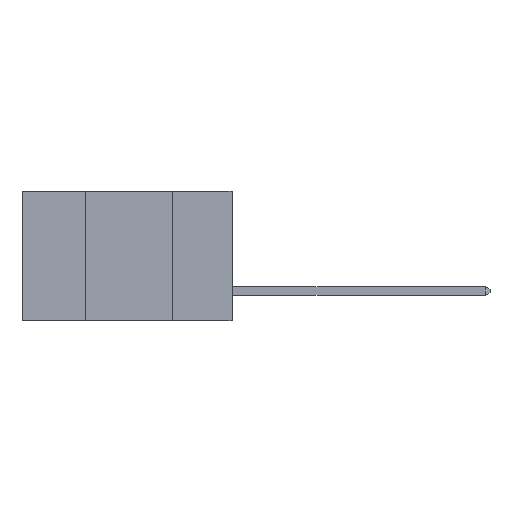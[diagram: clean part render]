
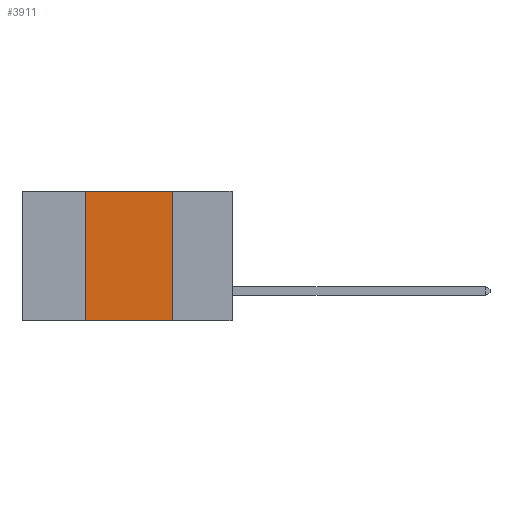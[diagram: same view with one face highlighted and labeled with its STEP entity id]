
A CAD part, left-side view. The second image highlights one B-rep face of the part: STEP entity #3911.
In plain terms, the highlighted planar face has unit normal (-1, 0, 0).
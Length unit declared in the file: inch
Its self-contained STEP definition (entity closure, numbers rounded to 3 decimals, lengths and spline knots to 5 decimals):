
#814 = VERTEX_POINT ( 'NONE', #1011 ) ;
#937 = CARTESIAN_POINT ( 'NONE',  ( 0., 0.42, -0.37 ) ) ;
#1011 = CARTESIAN_POINT ( 'NONE',  ( 0., 0.17, -0.37 ) ) ;
#1382 = VECTOR ( 'NONE', #5724, 39.37008 ) ;
#1448 = VERTEX_POINT ( 'NONE', #6835 ) ;
#3547 = VERTEX_POINT ( 'NONE', #10674 ) ;
#3552 = LINE ( 'NONE', #11912, #1382 ) ;
#3763 = FACE_OUTER_BOUND ( 'NONE', #13095, .T. ) ;
#3911 = ADVANCED_FACE ( 'NONE', ( #3763 ), #10203, .F. ) ;
#3932 = CARTESIAN_POINT ( 'NONE',  ( 0., 0.6, 0. ) ) ;
#3969 = CARTESIAN_POINT ( 'NONE',  ( 0., 0.17, 0. ) ) ;
#4545 = EDGE_CURVE ( 'NONE', #1448, #814, #10468, .T. ) ;
#4776 = LINE ( 'NONE', #7446, #13009 ) ;
#5025 = DIRECTION ( 'NONE',  ( 1., 0., 0. ) ) ;
#5724 = DIRECTION ( 'NONE',  ( 0., -1., 0. ) ) ;
#5783 = CARTESIAN_POINT ( 'NONE',  ( 0., 0.42, 0. ) ) ;
#5859 = ORIENTED_EDGE ( 'NONE', *, *, #4545, .F. ) ;
#6835 = CARTESIAN_POINT ( 'NONE',  ( 0., 0.17, 0. ) ) ;
#7157 = ORIENTED_EDGE ( 'NONE', *, *, #8226, .T. ) ;
#7313 = VECTOR ( 'NONE', #11976, 39.37008 ) ;
#7446 = CARTESIAN_POINT ( 'NONE',  ( 0., 0.6, -0.37 ) ) ;
#8134 = AXIS2_PLACEMENT_3D ( 'NONE', #3932, #5025, #12266 ) ;
#8226 = EDGE_CURVE ( 'NONE', #9420, #814, #4776, .T. ) ;
#9271 = ORIENTED_EDGE ( 'NONE', *, *, #12022, .F. ) ;
#9420 = VERTEX_POINT ( 'NONE', #937 ) ;
#9730 = EDGE_CURVE ( 'NONE', #3547, #1448, #3552, .T. ) ;
#10053 = LINE ( 'NONE', #5783, #7313 ) ;
#10203 = PLANE ( 'NONE',  #8134 ) ;
#10242 = DIRECTION ( 'NONE',  ( 0., 0., -1. ) ) ;
#10468 = LINE ( 'NONE', #3969, #12854 ) ;
#10674 = CARTESIAN_POINT ( 'NONE',  ( 0., 0.42, 0. ) ) ;
#11539 = DIRECTION ( 'NONE',  ( 0., -1., 0. ) ) ;
#11675 = ORIENTED_EDGE ( 'NONE', *, *, #9730, .F. ) ;
#11912 = CARTESIAN_POINT ( 'NONE',  ( 0., 0.6, 0. ) ) ;
#11976 = DIRECTION ( 'NONE',  ( 0., 0., 1. ) ) ;
#12022 = EDGE_CURVE ( 'NONE', #9420, #3547, #10053, .T. ) ;
#12266 = DIRECTION ( 'NONE',  ( 0., 0., -1. ) ) ;
#12854 = VECTOR ( 'NONE', #10242, 39.37008 ) ;
#13009 = VECTOR ( 'NONE', #11539, 39.37008 ) ;
#13095 = EDGE_LOOP ( 'NONE', ( #5859, #11675, #9271, #7157 ) ) ;
